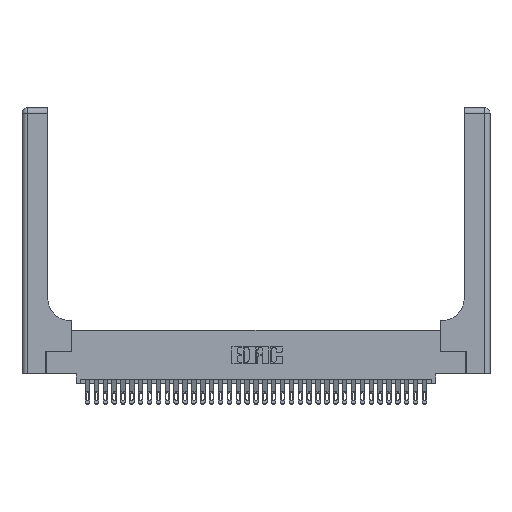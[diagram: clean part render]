
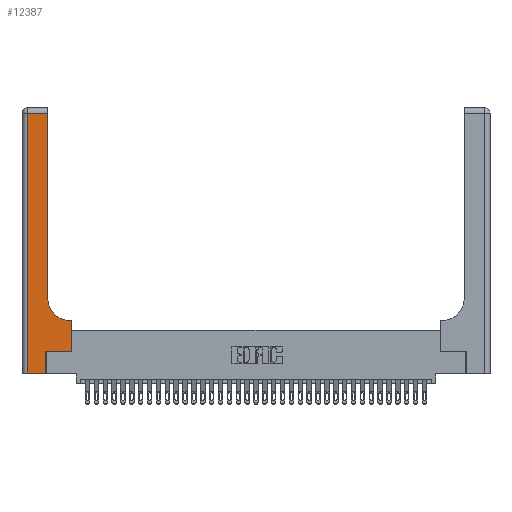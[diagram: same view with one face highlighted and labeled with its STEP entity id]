
A CAD part, top view. The second image highlights one B-rep face of the part: STEP entity #12387.
In plain terms, the highlighted planar face has unit normal (0, 0, 1).
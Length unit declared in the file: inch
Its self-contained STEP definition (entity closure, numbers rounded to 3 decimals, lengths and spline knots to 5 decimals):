
#1892 = CARTESIAN_POINT ( 'NONE',  ( 0., 2.94, 0.37 ) ) ;
#2456 = DIRECTION ( 'NONE',  ( -1., 0., 0. ) ) ;
#2567 = CARTESIAN_POINT ( 'NONE',  ( 0.5415, 0.85, 0.37 ) ) ;
#2613 = CARTESIAN_POINT ( 'NONE',  ( 0.2915, 3., 0.37 ) ) ;
#3184 = VERTEX_POINT ( 'NONE', #28463 ) ;
#3302 = ORIENTED_EDGE ( 'NONE', *, *, #24788, .T. ) ;
#4563 = ORIENTED_EDGE ( 'NONE', *, *, #17007, .T. ) ;
#4607 = ORIENTED_EDGE ( 'NONE', *, *, #26709, .T. ) ;
#4618 = VERTEX_POINT ( 'NONE', #32462 ) ;
#5008 = VERTEX_POINT ( 'NONE', #17479 ) ;
#5209 = VECTOR ( 'NONE', #27345, 39.37008 ) ;
#5395 = DIRECTION ( 'NONE',  ( 1., 0., 0. ) ) ;
#5415 = CARTESIAN_POINT ( 'NONE',  ( 0.5585, 0.25, 0.37 ) ) ;
#7123 = FACE_OUTER_BOUND ( 'NONE', #24195, .T. ) ;
#7319 = LINE ( 'NONE', #8624, #29893 ) ;
#8036 = CARTESIAN_POINT ( 'NONE',  ( 0., 0., 0.37 ) ) ;
#8086 = ORIENTED_EDGE ( 'NONE', *, *, #22173, .T. ) ;
#8211 = DIRECTION ( 'NONE',  ( 1., 0., 0. ) ) ;
#8624 = CARTESIAN_POINT ( 'NONE',  ( 0.06, 3., 0.37 ) ) ;
#8656 = EDGE_CURVE ( 'NONE', #20747, #31831, #13096, .T. ) ;
#9804 = CARTESIAN_POINT ( 'NONE',  ( 0.5585, 0.25, 0.37 ) ) ;
#10697 = AXIS2_PLACEMENT_3D ( 'NONE', #2567, #22317, #5395 ) ;
#10721 = DIRECTION ( 'NONE',  ( 0., 0., -1. ) ) ;
#11183 = VECTOR ( 'NONE', #2456, 39.37008 ) ;
#11537 = VERTEX_POINT ( 'NONE', #28695 ) ;
#12387 = ADVANCED_FACE ( 'NONE', ( #7123 ), #21973, .F. ) ;
#13096 = LINE ( 'NONE', #5415, #34760 ) ;
#13802 = VECTOR ( 'NONE', #23362, 39.37008 ) ;
#15662 = ORIENTED_EDGE ( 'NONE', *, *, #24638, .T. ) ;
#16528 = CARTESIAN_POINT ( 'NONE',  ( 0.2915, 0.6, 0.37 ) ) ;
#16780 = DIRECTION ( 'NONE',  ( 0., 1., 0. ) ) ;
#16974 = ORIENTED_EDGE ( 'NONE', *, *, #20357, .T. ) ;
#17007 = EDGE_CURVE ( 'NONE', #4618, #27015, #28947, .T. ) ;
#17404 = ORIENTED_EDGE ( 'NONE', *, *, #8656, .T. ) ;
#17443 = ORIENTED_EDGE ( 'NONE', *, *, #21562, .T. ) ;
#17479 = CARTESIAN_POINT ( 'NONE',  ( 0.06, 2.94, 0.37 ) ) ;
#17571 = LINE ( 'NONE', #8036, #23323 ) ;
#17855 = VECTOR ( 'NONE', #19516, 39.37008 ) ;
#18707 = LINE ( 'NONE', #16528, #11183 ) ;
#19174 = ORIENTED_EDGE ( 'NONE', *, *, #27188, .T. ) ;
#19516 = DIRECTION ( 'NONE',  ( 0., 1., 0. ) ) ;
#19661 = LINE ( 'NONE', #28006, #33807 ) ;
#20357 = EDGE_CURVE ( 'NONE', #24919, #11537, #25553, .T. ) ;
#20747 = VERTEX_POINT ( 'NONE', #9804 ) ;
#21562 = EDGE_CURVE ( 'NONE', #5008, #3184, #7319, .T. ) ;
#21973 = PLANE ( 'NONE',  #24996 ) ;
#22018 = LINE ( 'NONE', #1892, #5209 ) ;
#22173 = EDGE_CURVE ( 'NONE', #27015, #20747, #19661, .T. ) ;
#22317 = DIRECTION ( 'NONE',  ( 0., 0., -1. ) ) ;
#23323 = VECTOR ( 'NONE', #24983, 39.37008 ) ;
#23362 = DIRECTION ( 'NONE',  ( 0., 1., 0. ) ) ;
#24195 = EDGE_LOOP ( 'NONE', ( #4607, #15662, #17443, #3302, #4563, #8086, #17404, #19174, #16974 ) ) ;
#24327 = CARTESIAN_POINT ( 'NONE',  ( 0.269, 0.25, 0.37 ) ) ;
#24638 = EDGE_CURVE ( 'NONE', #28494, #5008, #22018, .T. ) ;
#24788 = EDGE_CURVE ( 'NONE', #3184, #4618, #17571, .T. ) ;
#24919 = VERTEX_POINT ( 'NONE', #34104 ) ;
#24983 = DIRECTION ( 'NONE',  ( 1., 0., 0. ) ) ;
#24996 = AXIS2_PLACEMENT_3D ( 'NONE', #27654, #10721, #30514 ) ;
#25365 = LINE ( 'NONE', #2613, #17855 ) ;
#25553 = CIRCLE ( 'NONE', #10697, 0.25 ) ;
#26709 = EDGE_CURVE ( 'NONE', #11537, #28494, #25365, .T. ) ;
#27015 = VERTEX_POINT ( 'NONE', #24327 ) ;
#27188 = EDGE_CURVE ( 'NONE', #31831, #24919, #18707, .T. ) ;
#27345 = DIRECTION ( 'NONE',  ( -1., 0., 0. ) ) ;
#27654 = CARTESIAN_POINT ( 'NONE',  ( 0., 3., 0.37 ) ) ;
#28006 = CARTESIAN_POINT ( 'NONE',  ( 0.269, 0.25, 0.37 ) ) ;
#28315 = CARTESIAN_POINT ( 'NONE',  ( 0.2915, 2.94, 0.37 ) ) ;
#28408 = DIRECTION ( 'NONE',  ( 0., -1., 0. ) ) ;
#28463 = CARTESIAN_POINT ( 'NONE',  ( 0.06, 0., 0.37 ) ) ;
#28494 = VERTEX_POINT ( 'NONE', #28315 ) ;
#28695 = CARTESIAN_POINT ( 'NONE',  ( 0.2915, 0.85, 0.37 ) ) ;
#28919 = CARTESIAN_POINT ( 'NONE',  ( 0.269, 0., 0.37 ) ) ;
#28947 = LINE ( 'NONE', #28919, #13802 ) ;
#29893 = VECTOR ( 'NONE', #28408, 39.37008 ) ;
#30514 = DIRECTION ( 'NONE',  ( -1., 0., 0. ) ) ;
#31831 = VERTEX_POINT ( 'NONE', #33601 ) ;
#32462 = CARTESIAN_POINT ( 'NONE',  ( 0.269, 0., 0.37 ) ) ;
#33601 = CARTESIAN_POINT ( 'NONE',  ( 0.5585, 0.6, 0.37 ) ) ;
#33807 = VECTOR ( 'NONE', #8211, 39.37008 ) ;
#34104 = CARTESIAN_POINT ( 'NONE',  ( 0.5415, 0.6, 0.37 ) ) ;
#34760 = VECTOR ( 'NONE', #16780, 39.37008 ) ;
